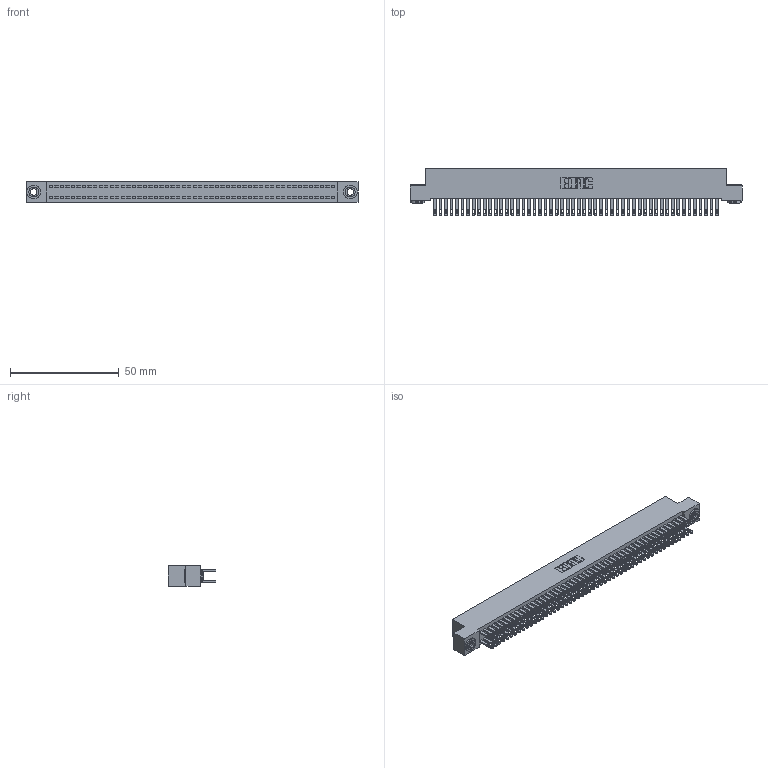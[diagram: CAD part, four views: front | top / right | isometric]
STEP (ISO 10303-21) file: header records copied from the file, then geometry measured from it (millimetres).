
FILE_DESCRIPTION (( 'STEP AP203' ), '1' );
FILE_NAME ('342-104-500-203.STEP', '2018-08-14T05:49:35', ( '' ), ( '' ), 'SwSTEP 2.0', 'SolidWorks 2016', '' );
FILE_SCHEMA (( 'CONFIG_CONTROL_DESIGN' ));
Length unit declared in the file: inch
Products named in the file (4): 342 Part_.156 TH; 345-292-001_345-293-100; 342-250-002_345-250-002-102; 342-104-500-203
Assembly tree (107 placements, depth 2):
  342-104-500-203
    342 Part_.156 TH
    345-292-001_345-293-100  x104
    342-250-002_345-250-002-102  x2
Bounding box: 152.4 x 21.85 x 9.4 mm (x, y, z)
Volume: 14081.1 mm3; surface area: 24376.7 mm2
Topology: 107 solids, 107 shells, 5140 faces, 15663 edges, 10438 vertices
Faces by surface type: plane 3196, cylinder 1936, cone 8
Entity records: 32608 total; most frequent: CARTESIAN_POINT 5365, ORIENTED_EDGE 5294, DIRECTION 4601, EDGE_CURVE 2647, LINE 2491, VECTOR 2491, VERTEX_POINT 1762, AXIS2_PLACEMENT_3D 1055
